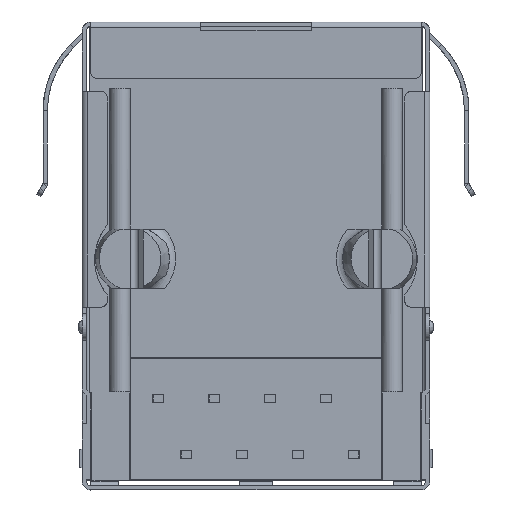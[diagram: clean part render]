
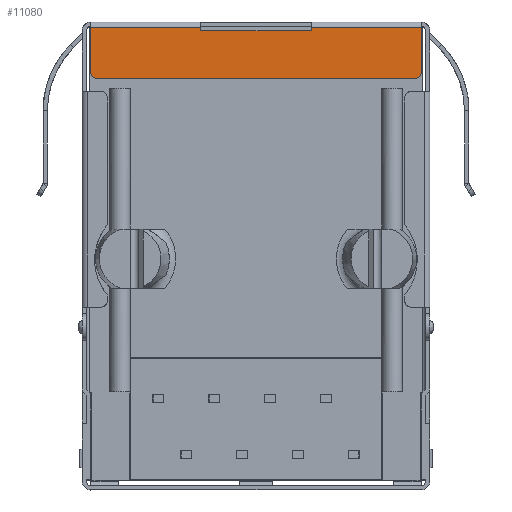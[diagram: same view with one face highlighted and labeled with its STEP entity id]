
A CAD part, front view. The second image highlights one B-rep face of the part: STEP entity #11080.
In plain terms, the highlighted planar face has unit normal (0, -1, 0).
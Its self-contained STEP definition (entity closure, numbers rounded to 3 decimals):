
#227 = DIRECTION ( 'NONE',  ( 0., 0., 1. ) ) ;
#1129 = DIRECTION ( 'NONE',  ( 1., 0., 0. ) ) ;
#1678 = EDGE_CURVE ( 'NONE', #32491, #18097, #26342, .T. ) ;
#2877 = CARTESIAN_POINT ( 'NONE',  ( 3.512, 6.085, 8.27 ) ) ;
#3177 = VECTOR ( 'NONE', #34551, 1000. ) ;
#3374 = CARTESIAN_POINT ( 'NONE',  ( -11.488, 6.085, 10.17 ) ) ;
#3897 = VERTEX_POINT ( 'NONE', #2877 ) ;
#4207 = LINE ( 'NONE', #14642, #38197 ) ;
#4709 = ORIENTED_EDGE ( 'NONE', *, *, #1678, .T. ) ;
#4804 = CIRCLE ( 'NONE', #39966, 0.25 ) ;
#4936 = CARTESIAN_POINT ( 'NONE',  ( -1.488, 6.085, 10.32 ) ) ;
#5268 = ORIENTED_EDGE ( 'NONE', *, *, #22826, .F. ) ;
#6317 = DIRECTION ( 'NONE',  ( 0., -1., 0. ) ) ;
#6447 = CARTESIAN_POINT ( 'NONE',  ( -11.238, 6.085, 8.02 ) ) ;
#6460 = CARTESIAN_POINT ( 'NONE',  ( 3.262, 6.085, 8.27 ) ) ;
#7857 = LINE ( 'NONE', #29198, #14038 ) ;
#8464 = CARTESIAN_POINT ( 'NONE',  ( -11.488, 6.085, 10.57 ) ) ;
#8509 = CARTESIAN_POINT ( 'NONE',  ( -11.238, 6.085, 8.27 ) ) ;
#8638 = CARTESIAN_POINT ( 'NONE',  ( -11.488, 6.085, 10.57 ) ) ;
#8949 = ORIENTED_EDGE ( 'NONE', *, *, #32479, .T. ) ;
#9554 = DIRECTION ( 'NONE',  ( 1., 0., 0. ) ) ;
#9864 = ORIENTED_EDGE ( 'NONE', *, *, #16636, .T. ) ;
#10545 = CARTESIAN_POINT ( 'NONE',  ( -11.488, 6.085, 10.32 ) ) ;
#10902 = CIRCLE ( 'NONE', #20369, 0.25 ) ;
#11080 = ADVANCED_FACE ( 'NONE', ( #42099 ), #35233, .T. ) ;
#11477 = DIRECTION ( 'NONE',  ( 0., 0., -1. ) ) ;
#11508 = VECTOR ( 'NONE', #40419, 1000. ) ;
#11594 = VECTOR ( 'NONE', #37988, 1000. ) ;
#11661 = CARTESIAN_POINT ( 'NONE',  ( -6.488, 6.085, 10.17 ) ) ;
#11811 = DIRECTION ( 'NONE',  ( 1., 0., 0. ) ) ;
#12489 = EDGE_LOOP ( 'NONE', ( #8949, #24018, #23359, #29504, #9864, #32359, #5268, #4709, #20357, #34483 ) ) ;
#12511 = VECTOR ( 'NONE', #11477, 1000. ) ;
#12680 = CARTESIAN_POINT ( 'NONE',  ( 3.262, 6.085, 8.02 ) ) ;
#12764 = CARTESIAN_POINT ( 'NONE',  ( -1.488, 6.085, 10.47 ) ) ;
#12815 = VECTOR ( 'NONE', #227, 1000. ) ;
#13663 = VERTEX_POINT ( 'NONE', #6447 ) ;
#14038 = VECTOR ( 'NONE', #9554, 1000. ) ;
#14039 = LINE ( 'NONE', #31530, #3177 ) ;
#14040 = CARTESIAN_POINT ( 'NONE',  ( 3.512, 6.085, 10.32 ) ) ;
#14642 = CARTESIAN_POINT ( 'NONE',  ( -11.488, 6.085, 8.02 ) ) ;
#16591 = CARTESIAN_POINT ( 'NONE',  ( -11.488, 6.085, 8.27 ) ) ;
#16636 = EDGE_CURVE ( 'NONE', #3897, #39735, #37260, .T. ) ;
#18097 = VERTEX_POINT ( 'NONE', #11661 ) ;
#20004 = VERTEX_POINT ( 'NONE', #16591 ) ;
#20303 = LINE ( 'NONE', #40922, #11594 ) ;
#20357 = ORIENTED_EDGE ( 'NONE', *, *, #37907, .T. ) ;
#20369 = AXIS2_PLACEMENT_3D ( 'NONE', #8509, #31499, #11811 ) ;
#22282 = VERTEX_POINT ( 'NONE', #4936 ) ;
#22826 = EDGE_CURVE ( 'NONE', #32491, #22282, #30782, .T. ) ;
#23359 = ORIENTED_EDGE ( 'NONE', *, *, #39334, .T. ) ;
#24002 = VERTEX_POINT ( 'NONE', #10545 ) ;
#24018 = ORIENTED_EDGE ( 'NONE', *, *, #34295, .T. ) ;
#25013 = AXIS2_PLACEMENT_3D ( 'NONE', #8638, #38270, #31765 ) ;
#25841 = DIRECTION ( 'NONE',  ( -1., 0., 0. ) ) ;
#26342 = LINE ( 'NONE', #3374, #38749 ) ;
#26360 = LINE ( 'NONE', #8464, #12511 ) ;
#29198 = CARTESIAN_POINT ( 'NONE',  ( -4.038, 6.085, 10.32 ) ) ;
#29504 = ORIENTED_EDGE ( 'NONE', *, *, #32201, .T. ) ;
#30782 = LINE ( 'NONE', #12764, #12815 ) ;
#31201 = EDGE_CURVE ( 'NONE', #24002, #36927, #20303, .T. ) ;
#31499 = DIRECTION ( 'NONE',  ( 0., -1., 0. ) ) ;
#31530 = CARTESIAN_POINT ( 'NONE',  ( -6.488, 6.085, 10.57 ) ) ;
#31765 = DIRECTION ( 'NONE',  ( 1., 0., 0. ) ) ;
#32201 = EDGE_CURVE ( 'NONE', #41605, #3897, #4804, .T. ) ;
#32359 = ORIENTED_EDGE ( 'NONE', *, *, #33071, .F. ) ;
#32479 = EDGE_CURVE ( 'NONE', #24002, #20004, #26360, .T. ) ;
#32491 = VERTEX_POINT ( 'NONE', #37926 ) ;
#32605 = CARTESIAN_POINT ( 'NONE',  ( -6.488, 6.085, 10.32 ) ) ;
#33071 = EDGE_CURVE ( 'NONE', #22282, #39735, #7857, .T. ) ;
#33445 = CARTESIAN_POINT ( 'NONE',  ( 3.512, 6.085, 10.57 ) ) ;
#34295 = EDGE_CURVE ( 'NONE', #20004, #13663, #10902, .T. ) ;
#34483 = ORIENTED_EDGE ( 'NONE', *, *, #31201, .F. ) ;
#34551 = DIRECTION ( 'NONE',  ( 0., 0., 1. ) ) ;
#35233 = PLANE ( 'NONE',  #25013 ) ;
#36927 = VERTEX_POINT ( 'NONE', #32605 ) ;
#37260 = LINE ( 'NONE', #33445, #11508 ) ;
#37907 = EDGE_CURVE ( 'NONE', #18097, #36927, #14039, .T. ) ;
#37926 = CARTESIAN_POINT ( 'NONE',  ( -1.488, 6.085, 10.17 ) ) ;
#37988 = DIRECTION ( 'NONE',  ( 1., 0., 0. ) ) ;
#38197 = VECTOR ( 'NONE', #1129, 1000. ) ;
#38270 = DIRECTION ( 'NONE',  ( 0., -1., 0. ) ) ;
#38749 = VECTOR ( 'NONE', #42717, 1000. ) ;
#39334 = EDGE_CURVE ( 'NONE', #13663, #41605, #4207, .T. ) ;
#39735 = VERTEX_POINT ( 'NONE', #14040 ) ;
#39966 = AXIS2_PLACEMENT_3D ( 'NONE', #6460, #6317, #25841 ) ;
#40419 = DIRECTION ( 'NONE',  ( 0., 0., 1. ) ) ;
#40922 = CARTESIAN_POINT ( 'NONE',  ( -3.938, 6.085, 10.32 ) ) ;
#41605 = VERTEX_POINT ( 'NONE', #12680 ) ;
#42099 = FACE_OUTER_BOUND ( 'NONE', #12489, .T. ) ;
#42717 = DIRECTION ( 'NONE',  ( -1., 0., 0. ) ) ;
